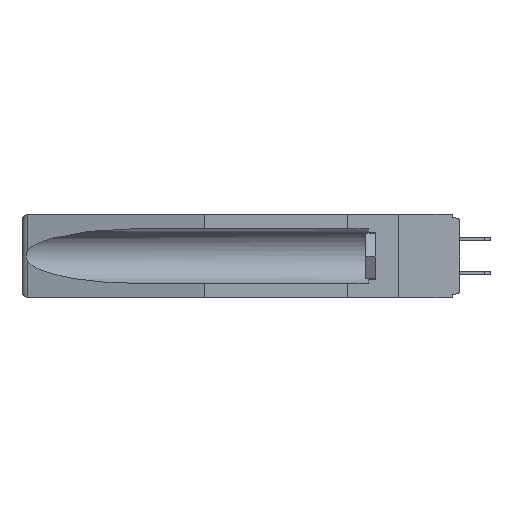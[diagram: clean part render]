
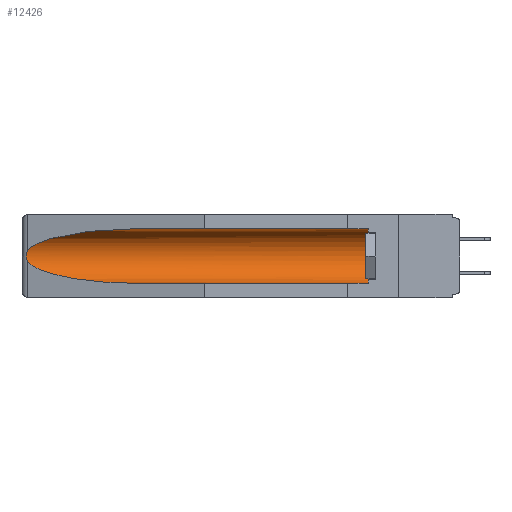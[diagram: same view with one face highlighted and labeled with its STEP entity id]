
A CAD part, left-side view. The second image highlights one B-rep face of the part: STEP entity #12426.
In plain terms, the highlighted cylindrical face has radius 2.857 mm (diameter 5.715 mm), a partial arc.
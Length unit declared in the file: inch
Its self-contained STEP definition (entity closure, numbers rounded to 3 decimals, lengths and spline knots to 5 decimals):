
#623 = DIRECTION ( 'NONE',  ( 0., 1., 0. ) ) ;
#1009 = CARTESIAN_POINT ( 'NONE',  ( 0.2673, 1.5327, -0.16383 ) ) ;
#1506 = VERTEX_POINT ( 'NONE', #14409 ) ;
#2086 = CARTESIAN_POINT ( 'NONE',  ( 0.155, 1.07973, -0.284 ) ) ;
#2814 = EDGE_CURVE ( 'NONE', #1506, #7979, #25339, .T. ) ;
#3199 = VERTEX_POINT ( 'NONE', #4307 ) ;
#3327 = EDGE_LOOP ( 'NONE', ( #15418, #25309, #20666, #19045, #12529, #21698 ) ) ;
#3660 = EDGE_CURVE ( 'NONE', #7979, #6388, #6549, .T. ) ;
#4148 = CARTESIAN_POINT ( 'NONE',  ( 0.26537, 1.52718, -0.19328 ) ) ;
#4307 = CARTESIAN_POINT ( 'NONE',  ( 0.155, 0.126, -0.284 ) ) ;
#4312 = CARTESIAN_POINT ( 'NONE',  ( 0.155, -0.30754, -0.284 ) ) ;
#5492 = CARTESIAN_POINT ( 'NONE',  ( 0.2675, 1.53308, -0.16763 ) ) ;
#6353 = EDGE_CURVE ( 'NONE', #6388, #9754, #24279, .T. ) ;
#6388 = VERTEX_POINT ( 'NONE', #22276 ) ;
#6549 =( BOUNDED_CURVE ( )  B_SPLINE_CURVE ( 3, ( #25003, #14553, #20920, #22975 ),
 .UNSPECIFIED., .F., .F. ) 
 B_SPLINE_CURVE_WITH_KNOTS ( ( 4, 4 ),
 ( 4.71239, 6.08839 ),
 .UNSPECIFIED. ) 
 CURVE ( )  GEOMETRIC_REPRESENTATION_ITEM ( )  RATIONAL_B_SPLINE_CURVE ( ( 1., 0.848, 0.848, 1. ) ) 
 REPRESENTATION_ITEM ( '' )  );
#6924 = CYLINDRICAL_SURFACE ( 'NONE', #17361, 0.1125 ) ;
#7439 = DIRECTION ( 'NONE',  ( 0., 1., 0. ) ) ;
#7979 = VERTEX_POINT ( 'NONE', #16002 ) ;
#9565 = DIRECTION ( 'NONE',  ( 0., 1., 0. ) ) ;
#9754 = VERTEX_POINT ( 'NONE', #15010 ) ;
#9773 = CARTESIAN_POINT ( 'NONE',  ( 0.26654, 1.53092, -0.15636 ) ) ;
#10913 = AXIS2_PLACEMENT_3D ( 'NONE', #22057, #24537, #19993 ) ;
#11340 = EDGE_CURVE ( 'NONE', #3199, #14614, #19419, .T. ) ;
#11830 = CARTESIAN_POINT ( 'NONE',  ( 0.26655, 1.53094, -0.18657 ) ) ;
#12422 = FACE_OUTER_BOUND ( 'NONE', #3327, .T. ) ;
#12426 = ADVANCED_FACE ( 'NONE', ( #12422 ), #6924, .F. ) ;
#12529 = ORIENTED_EDGE ( 'NONE', *, *, #17471, .T. ) ;
#13810 = CARTESIAN_POINT ( 'NONE',  ( 0.155, -0.30754, -0.1715 ) ) ;
#13908 = CIRCLE ( 'NONE', #10913, 0.1125 ) ;
#14409 = CARTESIAN_POINT ( 'NONE',  ( 0.155, 0.126, -0.059 ) ) ;
#14553 = CARTESIAN_POINT ( 'NONE',  ( 0.21114, 1.30732, -0.059 ) ) ;
#14614 = VERTEX_POINT ( 'NONE', #17108 ) ;
#15010 = CARTESIAN_POINT ( 'NONE',  ( 0.26537, 1.52718, -0.19328 ) ) ;
#15418 = ORIENTED_EDGE ( 'NONE', *, *, #3660, .T. ) ;
#15780 = VECTOR ( 'NONE', #623, 39.37008 ) ;
#15876 = CARTESIAN_POINT ( 'NONE',  ( 0.26597, 1.52961, -0.15275 ) ) ;
#16002 = CARTESIAN_POINT ( 'NONE',  ( 0.155, 1.07973, -0.059 ) ) ;
#16336 = VECTOR ( 'NONE', #9565, 39.37008 ) ;
#17108 = CARTESIAN_POINT ( 'NONE',  ( 0.155, 1.07973, -0.284 ) ) ;
#17361 = AXIS2_PLACEMENT_3D ( 'NONE', #13810, #7439, #24533 ) ;
#17471 = EDGE_CURVE ( 'NONE', #3199, #1506, #13908, .T. ) ;
#17991 = CARTESIAN_POINT ( 'NONE',  ( 0.26537, 1.52718, -0.19328 ) ) ;
#19045 = ORIENTED_EDGE ( 'NONE', *, *, #11340, .F. ) ;
#19419 = LINE ( 'NONE', #4312, #15780 ) ;
#19993 = DIRECTION ( 'NONE',  ( 0., 0., 1. ) ) ;
#20209 = CARTESIAN_POINT ( 'NONE',  ( 0.2675, 1.53308, -0.17534 ) ) ;
#20406 = CARTESIAN_POINT ( 'NONE',  ( 0.2673, 1.53269, -0.17917 ) ) ;
#20666 = ORIENTED_EDGE ( 'NONE', *, *, #23671, .T. ) ;
#20920 = CARTESIAN_POINT ( 'NONE',  ( 0.25451, 1.48313, -0.09465 ) ) ;
#21093 = CARTESIAN_POINT ( 'NONE',  ( 0.25451, 1.48313, -0.24835 ) ) ;
#21292 = CARTESIAN_POINT ( 'NONE',  ( 0.155, -0.30754, -0.059 ) ) ;
#21698 = ORIENTED_EDGE ( 'NONE', *, *, #2814, .T. ) ;
#22057 = CARTESIAN_POINT ( 'NONE',  ( 0.155, 0.126, -0.1715 ) ) ;
#22276 = CARTESIAN_POINT ( 'NONE',  ( 0.26537, 1.52718, -0.14972 ) ) ;
#22975 = CARTESIAN_POINT ( 'NONE',  ( 0.26537, 1.52718, -0.14972 ) ) ;
#23671 = EDGE_CURVE ( 'NONE', #9754, #14614, #27331, .T. ) ;
#24279 = B_SPLINE_CURVE_WITH_KNOTS ( 'NONE', 3,
 ( #24403, #15876, #9773, #1009, #5492, #20209, #20406, #11830, #26628, #17991 ),
 .UNSPECIFIED., .F., .F.,
 ( 4, 2, 2, 2, 4 ),
 ( 0., 0.00029, 0.00058, 0.00087, 0.00117 ),
 .UNSPECIFIED. ) ;
#24403 = CARTESIAN_POINT ( 'NONE',  ( 0.26537, 1.52718, -0.14972 ) ) ;
#24533 = DIRECTION ( 'NONE',  ( 0., 0., 1. ) ) ;
#24537 = DIRECTION ( 'NONE',  ( 0., -1., 0. ) ) ;
#25003 = CARTESIAN_POINT ( 'NONE',  ( 0.155, 1.07973, -0.059 ) ) ;
#25309 = ORIENTED_EDGE ( 'NONE', *, *, #6353, .T. ) ;
#25339 = LINE ( 'NONE', #21292, #16336 ) ;
#26628 = CARTESIAN_POINT ( 'NONE',  ( 0.26597, 1.5296, -0.19026 ) ) ;
#27331 =( BOUNDED_CURVE ( )  B_SPLINE_CURVE ( 3, ( #4148, #21093, #27405, #2086 ),
 .UNSPECIFIED., .F., .F. ) 
 B_SPLINE_CURVE_WITH_KNOTS ( ( 4, 4 ),
 ( 0.1948, 1.5708 ),
 .UNSPECIFIED. ) 
 CURVE ( )  GEOMETRIC_REPRESENTATION_ITEM ( )  RATIONAL_B_SPLINE_CURVE ( ( 1., 0.848, 0.848, 1. ) ) 
 REPRESENTATION_ITEM ( '' )  );
#27405 = CARTESIAN_POINT ( 'NONE',  ( 0.21114, 1.30732, -0.284 ) ) ;
